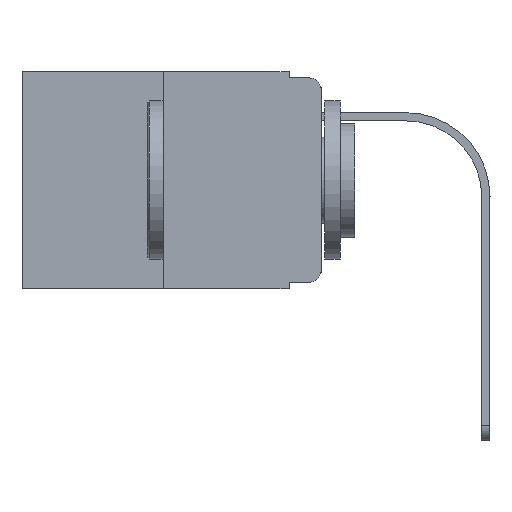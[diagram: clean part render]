
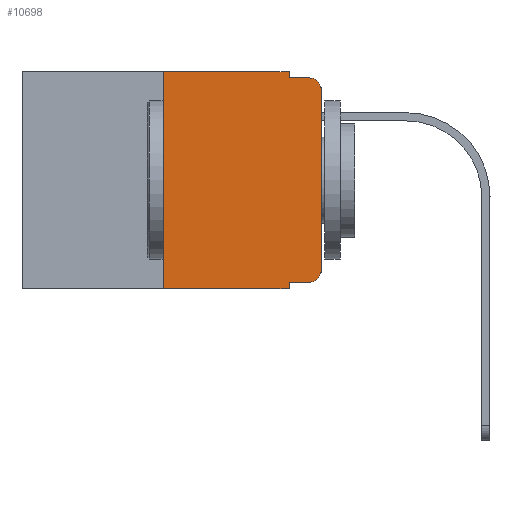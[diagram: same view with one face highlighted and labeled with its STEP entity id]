
A CAD part, left-side view. The second image highlights one B-rep face of the part: STEP entity #10698.
In plain terms, the highlighted planar face has unit normal (-1, 0, 0).
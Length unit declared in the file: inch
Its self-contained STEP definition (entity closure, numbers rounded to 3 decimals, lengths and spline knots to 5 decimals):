
#4 = CARTESIAN_POINT ( 'NONE',  ( 0., 0., 0. ) ) ;
#73 = CARTESIAN_POINT ( 'NONE',  ( 0., 0.051, -0.333 ) ) ;
#541 = CARTESIAN_POINT ( 'NONE',  ( 0., 0.473, 0. ) ) ;
#544 = CARTESIAN_POINT ( 'NONE',  ( 0., 0.473, -0.343 ) ) ;
#566 = VERTEX_POINT ( 'NONE', #6836 ) ;
#861 = EDGE_CURVE ( 'NONE', #5207, #4340, #12143, .T. ) ;
#913 = EDGE_CURVE ( 'NONE', #566, #4076, #5531, .T. ) ;
#1185 = ORIENTED_EDGE ( 'NONE', *, *, #913, .F. ) ;
#1203 = ORIENTED_EDGE ( 'NONE', *, *, #7998, .F. ) ;
#1211 = FACE_OUTER_BOUND ( 'NONE', #3533, .T. ) ;
#1370 = VECTOR ( 'NONE', #11290, 39.37008 ) ;
#1481 = EDGE_CURVE ( 'NONE', #8744, #5955, #10459, .T. ) ;
#1667 = VERTEX_POINT ( 'NONE', #9698 ) ;
#1765 = DIRECTION ( 'NONE',  ( 0., 0., -1. ) ) ;
#1825 = CARTESIAN_POINT ( 'NONE',  ( 0., 0.051, 0. ) ) ;
#1866 = CARTESIAN_POINT ( 'NONE',  ( 0., 0.02, -0.01 ) ) ;
#1941 = DIRECTION ( 'NONE',  ( 0., 0., 1. ) ) ;
#1946 = DIRECTION ( 'NONE',  ( 0., -1., 0. ) ) ;
#2164 = DIRECTION ( 'NONE',  ( 0., 0., -1. ) ) ;
#2571 = VERTEX_POINT ( 'NONE', #10592 ) ;
#2596 = VECTOR ( 'NONE', #10875, 39.37008 ) ;
#2637 = AXIS2_PLACEMENT_3D ( 'NONE', #8571, #5737, #6655 ) ;
#2964 = VECTOR ( 'NONE', #4624, 39.37008 ) ;
#3094 = LINE ( 'NONE', #8901, #6965 ) ;
#3136 = ORIENTED_EDGE ( 'NONE', *, *, #4855, .F. ) ;
#3211 = DIRECTION ( 'NONE',  ( 0., 0., -1. ) ) ;
#3438 = LINE ( 'NONE', #541, #3842 ) ;
#3533 = EDGE_LOOP ( 'NONE', ( #3877, #3771, #1185, #11208, #3136, #12067, #9703, #1203, #10614, #11443 ) ) ;
#3764 = AXIS2_PLACEMENT_3D ( 'NONE', #8260, #7518, #7330 ) ;
#3771 = ORIENTED_EDGE ( 'NONE', *, *, #9341, .T. ) ;
#3842 = VECTOR ( 'NONE', #7211, 39.37008 ) ;
#3877 = ORIENTED_EDGE ( 'NONE', *, *, #1481, .T. ) ;
#4076 = VERTEX_POINT ( 'NONE', #1866 ) ;
#4340 = VERTEX_POINT ( 'NONE', #7791 ) ;
#4624 = DIRECTION ( 'NONE',  ( 0., 0., 1. ) ) ;
#4855 = EDGE_CURVE ( 'NONE', #1667, #2571, #3438, .T. ) ;
#5046 = VECTOR ( 'NONE', #1941, 39.37008 ) ;
#5207 = VERTEX_POINT ( 'NONE', #8808 ) ;
#5258 = CARTESIAN_POINT ( 'NONE',  ( 0., 0., -0.313 ) ) ;
#5422 = LINE ( 'NONE', #1825, #6354 ) ;
#5501 = VERTEX_POINT ( 'NONE', #6395 ) ;
#5531 = LINE ( 'NONE', #10410, #6901 ) ;
#5737 = DIRECTION ( 'NONE',  ( 1., 0., 0. ) ) ;
#5955 = VERTEX_POINT ( 'NONE', #10316 ) ;
#6065 = CARTESIAN_POINT ( 'NONE',  ( 0., 0.02, -0.313 ) ) ;
#6128 = VERTEX_POINT ( 'NONE', #6724 ) ;
#6298 = LINE ( 'NONE', #544, #2596 ) ;
#6354 = VECTOR ( 'NONE', #1765, 39.37008 ) ;
#6395 = CARTESIAN_POINT ( 'NONE',  ( 0., 0.051, -0.343 ) ) ;
#6482 = CARTESIAN_POINT ( 'NONE',  ( 0., 0.25, 0. ) ) ;
#6655 = DIRECTION ( 'NONE',  ( 0., 0., -1. ) ) ;
#6724 = CARTESIAN_POINT ( 'NONE',  ( 0., 0.25, -0.343 ) ) ;
#6836 = CARTESIAN_POINT ( 'NONE',  ( 0., 0.051, -0.01 ) ) ;
#6901 = VECTOR ( 'NONE', #1946, 39.37008 ) ;
#6965 = VECTOR ( 'NONE', #2164, 39.37008 ) ;
#7211 = DIRECTION ( 'NONE',  ( 0., -1., 0. ) ) ;
#7330 = DIRECTION ( 'NONE',  ( 0., 0., -1. ) ) ;
#7518 = DIRECTION ( 'NONE',  ( -1., 0., 0. ) ) ;
#7791 = CARTESIAN_POINT ( 'NONE',  ( 0., 0.02, -0.333 ) ) ;
#7998 = EDGE_CURVE ( 'NONE', #5207, #5501, #5422, .T. ) ;
#8260 = CARTESIAN_POINT ( 'NONE',  ( 0., 0.02, -0.03 ) ) ;
#8533 = AXIS2_PLACEMENT_3D ( 'NONE', #6065, #10567, #3211 ) ;
#8571 = CARTESIAN_POINT ( 'NONE',  ( 0., 0.473, 0. ) ) ;
#8744 = VERTEX_POINT ( 'NONE', #5258 ) ;
#8808 = CARTESIAN_POINT ( 'NONE',  ( 0., 0.051, -0.333 ) ) ;
#8901 = CARTESIAN_POINT ( 'NONE',  ( 0., 0.051, 0. ) ) ;
#9258 = EDGE_CURVE ( 'NONE', #6128, #5501, #6298, .T. ) ;
#9341 = EDGE_CURVE ( 'NONE', #5955, #4076, #9502, .T. ) ;
#9502 = CIRCLE ( 'NONE', #3764, 0.02 ) ;
#9698 = CARTESIAN_POINT ( 'NONE',  ( 0., 0.25, 0. ) ) ;
#9703 = ORIENTED_EDGE ( 'NONE', *, *, #9258, .T. ) ;
#10316 = CARTESIAN_POINT ( 'NONE',  ( 0., 0., -0.03 ) ) ;
#10410 = CARTESIAN_POINT ( 'NONE',  ( 0., 0.051, -0.01 ) ) ;
#10459 = LINE ( 'NONE', #4, #5046 ) ;
#10567 = DIRECTION ( 'NONE',  ( -1., 0., 0. ) ) ;
#10592 = CARTESIAN_POINT ( 'NONE',  ( 0., 0.051, 0. ) ) ;
#10611 = PLANE ( 'NONE',  #2637 ) ;
#10614 = ORIENTED_EDGE ( 'NONE', *, *, #861, .T. ) ;
#10635 = EDGE_CURVE ( 'NONE', #6128, #1667, #11066, .T. ) ;
#10698 = ADVANCED_FACE ( 'NONE', ( #1211 ), #10611, .F. ) ;
#10707 = CIRCLE ( 'NONE', #8533, 0.02 ) ;
#10875 = DIRECTION ( 'NONE',  ( 0., -1., 0. ) ) ;
#11066 = LINE ( 'NONE', #6482, #2964 ) ;
#11208 = ORIENTED_EDGE ( 'NONE', *, *, #12212, .F. ) ;
#11290 = DIRECTION ( 'NONE',  ( 0., -1., 0. ) ) ;
#11443 = ORIENTED_EDGE ( 'NONE', *, *, #12128, .T. ) ;
#12067 = ORIENTED_EDGE ( 'NONE', *, *, #10635, .F. ) ;
#12128 = EDGE_CURVE ( 'NONE', #4340, #8744, #10707, .T. ) ;
#12143 = LINE ( 'NONE', #73, #1370 ) ;
#12212 = EDGE_CURVE ( 'NONE', #2571, #566, #3094, .T. ) ;
